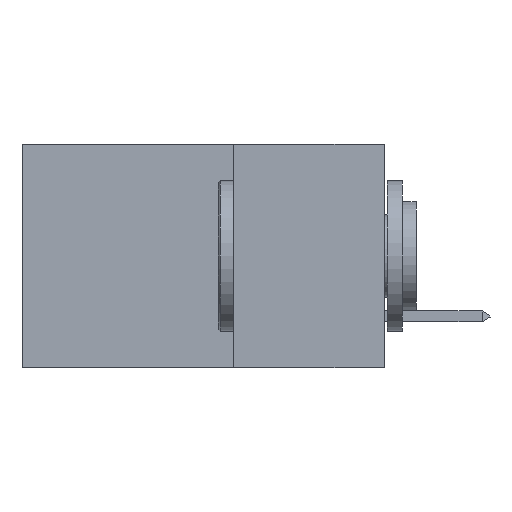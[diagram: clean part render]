
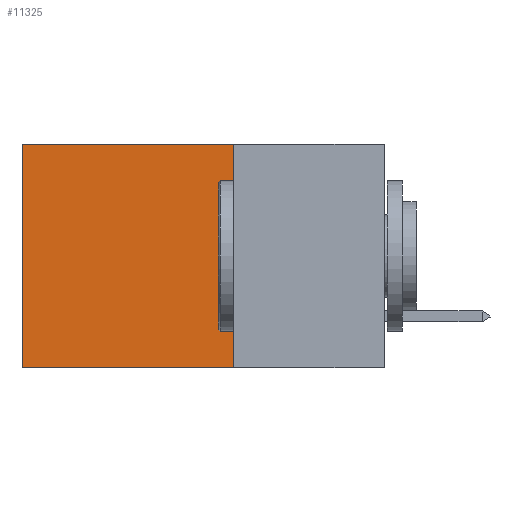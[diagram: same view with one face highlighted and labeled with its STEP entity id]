
A CAD part, left-side view. The second image highlights one B-rep face of the part: STEP entity #11325.
In plain terms, the highlighted planar face has unit normal (-1, 0, 0).
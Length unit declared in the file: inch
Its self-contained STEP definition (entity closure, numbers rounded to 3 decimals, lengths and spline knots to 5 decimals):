
#231 = FACE_OUTER_BOUND ( 'NONE', #21148, .T. ) ;
#286 = VECTOR ( 'NONE', #13741, 39.37008 ) ;
#550 = DIRECTION ( 'NONE',  ( 0., 0., -1. ) ) ;
#1578 = VECTOR ( 'NONE', #4868, 39.37008 ) ;
#3606 = CARTESIAN_POINT ( 'NONE',  ( 0.2875, 0.25, 0. ) ) ;
#3804 = LINE ( 'NONE', #7789, #286 ) ;
#3877 = ORIENTED_EDGE ( 'NONE', *, *, #18550, .T. ) ;
#4868 = DIRECTION ( 'NONE',  ( 0., 1., 0. ) ) ;
#4876 = DIRECTION ( 'NONE',  ( 0., 1., 0. ) ) ;
#5196 = LINE ( 'NONE', #15030, #17174 ) ;
#5293 = EDGE_CURVE ( 'NONE', #12720, #6012, #17044, .T. ) ;
#5449 = ORIENTED_EDGE ( 'NONE', *, *, #9548, .F. ) ;
#6012 = VERTEX_POINT ( 'NONE', #23893 ) ;
#6900 = CARTESIAN_POINT ( 'NONE',  ( 0.2875, 0.25, 0. ) ) ;
#7105 = CARTESIAN_POINT ( 'NONE',  ( 0.2875, 0.6, 0. ) ) ;
#7789 = CARTESIAN_POINT ( 'NONE',  ( 0.2875, 0.6, 0. ) ) ;
#8170 = CARTESIAN_POINT ( 'NONE',  ( 0.2875, 0.25, 0. ) ) ;
#9548 = EDGE_CURVE ( 'NONE', #6012, #16312, #5196, .T. ) ;
#9782 = VERTEX_POINT ( 'NONE', #7105 ) ;
#10099 = CARTESIAN_POINT ( 'NONE',  ( 0.2875, 0.6, -0.37 ) ) ;
#10784 = CARTESIAN_POINT ( 'NONE',  ( 0.2875, 0.25, 0. ) ) ;
#10873 = EDGE_CURVE ( 'NONE', #9782, #16312, #3804, .T. ) ;
#11325 = ADVANCED_FACE ( 'NONE', ( #231 ), #12244, .F. ) ;
#12244 = PLANE ( 'NONE',  #17678 ) ;
#12720 = VERTEX_POINT ( 'NONE', #8170 ) ;
#13741 = DIRECTION ( 'NONE',  ( 0., 0., -1. ) ) ;
#15030 = CARTESIAN_POINT ( 'NONE',  ( 0.2875, 0.25, -0.37 ) ) ;
#16282 = DIRECTION ( 'NONE',  ( 1., 0., 0. ) ) ;
#16312 = VERTEX_POINT ( 'NONE', #10099 ) ;
#17044 = LINE ( 'NONE', #6900, #24847 ) ;
#17174 = VECTOR ( 'NONE', #4876, 39.37008 ) ;
#17409 = LINE ( 'NONE', #10784, #1578 ) ;
#17678 = AXIS2_PLACEMENT_3D ( 'NONE', #3606, #16282, #18239 ) ;
#18239 = DIRECTION ( 'NONE',  ( 0., 0., -1. ) ) ;
#18550 = EDGE_CURVE ( 'NONE', #12720, #9782, #17409, .T. ) ;
#21148 = EDGE_LOOP ( 'NONE', ( #22485, #5449, #21946, #3877 ) ) ;
#21946 = ORIENTED_EDGE ( 'NONE', *, *, #5293, .F. ) ;
#22485 = ORIENTED_EDGE ( 'NONE', *, *, #10873, .T. ) ;
#23893 = CARTESIAN_POINT ( 'NONE',  ( 0.2875, 0.25, -0.37 ) ) ;
#24847 = VECTOR ( 'NONE', #550, 39.37008 ) ;
